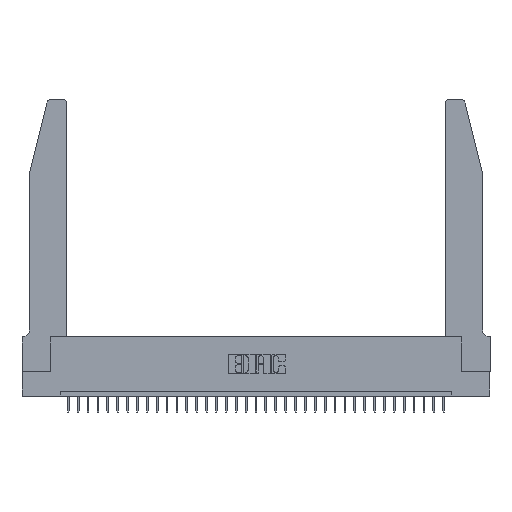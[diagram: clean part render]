
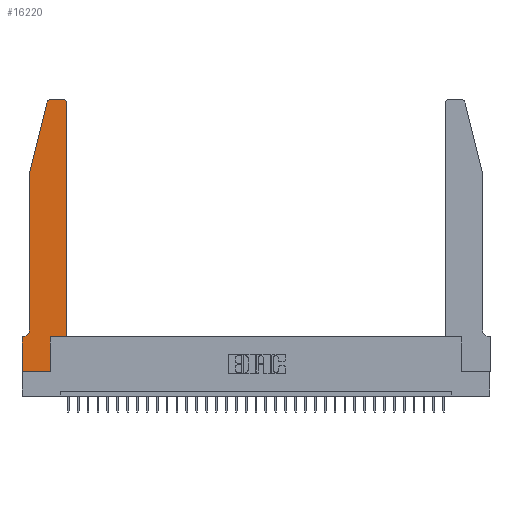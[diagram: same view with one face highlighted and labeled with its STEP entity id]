
A CAD part, top view. The second image highlights one B-rep face of the part: STEP entity #16220.
In plain terms, the highlighted planar face has unit normal (0, 0, 1).
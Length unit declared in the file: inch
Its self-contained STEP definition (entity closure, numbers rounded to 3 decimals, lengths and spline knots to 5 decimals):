
#76 = LINE ( 'NONE', #32654, #25574 ) ;
#505 = LINE ( 'NONE', #14812, #14825 ) ;
#1436 = ORIENTED_EDGE ( 'NONE', *, *, #25643, .T. ) ;
#1445 = ORIENTED_EDGE ( 'NONE', *, *, #2100, .T. ) ;
#1722 = LINE ( 'NONE', #32258, #25044 ) ;
#1838 = CARTESIAN_POINT ( 'NONE',  ( 0.0755, 0.42, 0.37 ) ) ;
#2100 = EDGE_CURVE ( 'NONE', #6404, #25170, #1722, .T. ) ;
#2389 = CIRCLE ( 'NONE', #14596, 0.03 ) ;
#2399 = CARTESIAN_POINT ( 'NONE',  ( 0.0755, 0.35, 0.37 ) ) ;
#2851 = ORIENTED_EDGE ( 'NONE', *, *, #15162, .T. ) ;
#3322 = EDGE_LOOP ( 'NONE', ( #1445, #31529, #28126, #1436, #2851, #7869, #8199, #13183, #10939, #4175, #20992, #10540 ) ) ;
#3427 = LINE ( 'NONE', #25641, #8886 ) ;
#3844 = CARTESIAN_POINT ( 'NONE',  ( 0.2865, 0., 0.37 ) ) ;
#3898 = FACE_OUTER_BOUND ( 'NONE', #3322, .T. ) ;
#4175 = ORIENTED_EDGE ( 'NONE', *, *, #10695, .T. ) ;
#4227 = DIRECTION ( 'NONE',  ( 0., -1., 0. ) ) ;
#4323 = VECTOR ( 'NONE', #4227, 39.37008 ) ;
#4511 = AXIS2_PLACEMENT_3D ( 'NONE', #9586, #7115, #20034 ) ;
#4575 = VERTEX_POINT ( 'NONE', #20891 ) ;
#6296 = CARTESIAN_POINT ( 'NONE',  ( 0.0755, 2., 0.37 ) ) ;
#6371 = VECTOR ( 'NONE', #29928, 39.37008 ) ;
#6404 = VERTEX_POINT ( 'NONE', #23749 ) ;
#7115 = DIRECTION ( 'NONE',  ( 0., 0., 1. ) ) ;
#7869 = ORIENTED_EDGE ( 'NONE', *, *, #23926, .T. ) ;
#8017 = EDGE_CURVE ( 'NONE', #28567, #26622, #76, .T. ) ;
#8063 = CARTESIAN_POINT ( 'NONE',  ( 0.4505, 0.35, 0.37 ) ) ;
#8086 = EDGE_CURVE ( 'NONE', #15128, #24139, #9329, .T. ) ;
#8184 = EDGE_CURVE ( 'NONE', #10328, #4575, #3427, .T. ) ;
#8199 = ORIENTED_EDGE ( 'NONE', *, *, #8086, .T. ) ;
#8257 = VERTEX_POINT ( 'NONE', #1838 ) ;
#8379 = CIRCLE ( 'NONE', #16040, 0.03 ) ;
#8787 = VECTOR ( 'NONE', #34493, 39.37008 ) ;
#8886 = VECTOR ( 'NONE', #15410, 39.37008 ) ;
#9039 = DIRECTION ( 'NONE',  ( 0., 0., -1. ) ) ;
#9090 = EDGE_CURVE ( 'NONE', #26622, #6404, #8379, .T. ) ;
#9329 = LINE ( 'NONE', #17511, #4323 ) ;
#9586 = CARTESIAN_POINT ( 'NONE',  ( 0., 0.35, 0.37 ) ) ;
#10328 = VERTEX_POINT ( 'NONE', #3844 ) ;
#10430 = CARTESIAN_POINT ( 'NONE',  ( 0.284, 2.75, 0.37 ) ) ;
#10540 = ORIENTED_EDGE ( 'NONE', *, *, #9090, .T. ) ;
#10667 = CIRCLE ( 'NONE', #18824, 0.07 ) ;
#10695 = EDGE_CURVE ( 'NONE', #4575, #28567, #12264, .T. ) ;
#10939 = ORIENTED_EDGE ( 'NONE', *, *, #8184, .T. ) ;
#11753 = CARTESIAN_POINT ( 'NONE',  ( 0.25487, 2.72718, 0.37 ) ) ;
#12174 = CARTESIAN_POINT ( 'NONE',  ( 0.284, 2.72, 0.37 ) ) ;
#12241 = DIRECTION ( 'NONE',  ( 1., 0., 0. ) ) ;
#12264 = LINE ( 'NONE', #8063, #6371 ) ;
#13183 = ORIENTED_EDGE ( 'NONE', *, *, #15821, .T. ) ;
#13275 = DIRECTION ( 'NONE',  ( -0.239, -0.971, 0. ) ) ;
#13540 = CARTESIAN_POINT ( 'NONE',  ( 0., 0., 0.37 ) ) ;
#13716 = EDGE_CURVE ( 'NONE', #25170, #24223, #2389, .T. ) ;
#13723 = LINE ( 'NONE', #6296, #27377 ) ;
#13868 = DIRECTION ( 'NONE',  ( 0., 0., 1. ) ) ;
#14596 = AXIS2_PLACEMENT_3D ( 'NONE', #12174, #30669, #25151 ) ;
#14812 = CARTESIAN_POINT ( 'NONE',  ( 0., 0., 0.37 ) ) ;
#14825 = VECTOR ( 'NONE', #12241, 39.37008 ) ;
#15128 = VERTEX_POINT ( 'NONE', #33172 ) ;
#15162 = EDGE_CURVE ( 'NONE', #8257, #18800, #10667, .T. ) ;
#15410 = DIRECTION ( 'NONE',  ( 0., 1., 0. ) ) ;
#15821 = EDGE_CURVE ( 'NONE', #24139, #10328, #505, .T. ) ;
#15838 = EDGE_CURVE ( 'NONE', #24223, #34137, #31050, .T. ) ;
#16040 = AXIS2_PLACEMENT_3D ( 'NONE', #29435, #13868, #16638 ) ;
#16220 = ADVANCED_FACE ( 'NONE', ( #3898 ), #23061, .T. ) ;
#16638 = DIRECTION ( 'NONE',  ( 1., 0., 0. ) ) ;
#16772 = DIRECTION ( 'NONE',  ( 0., -1., 0. ) ) ;
#17511 = CARTESIAN_POINT ( 'NONE',  ( 0., 0., 0.37 ) ) ;
#18785 = LINE ( 'NONE', #2399, #8787 ) ;
#18800 = VERTEX_POINT ( 'NONE', #33409 ) ;
#18824 = AXIS2_PLACEMENT_3D ( 'NONE', #30354, #9039, #27759 ) ;
#19197 = DIRECTION ( 'NONE',  ( 0., 1., 0. ) ) ;
#19627 = CARTESIAN_POINT ( 'NONE',  ( 0.4505, 0.35, 0.37 ) ) ;
#20034 = DIRECTION ( 'NONE',  ( 1., 0., 0. ) ) ;
#20183 = VECTOR ( 'NONE', #13275, 39.37008 ) ;
#20891 = CARTESIAN_POINT ( 'NONE',  ( 0.2865, 0.35, 0.37 ) ) ;
#20992 = ORIENTED_EDGE ( 'NONE', *, *, #8017, .T. ) ;
#22670 = CARTESIAN_POINT ( 'NONE',  ( 0.0755, 2., 0.37 ) ) ;
#23061 = PLANE ( 'NONE',  #4511 ) ;
#23749 = CARTESIAN_POINT ( 'NONE',  ( 0.4205, 2.75, 0.37 ) ) ;
#23926 = EDGE_CURVE ( 'NONE', #18800, #15128, #18785, .T. ) ;
#24139 = VERTEX_POINT ( 'NONE', #13540 ) ;
#24223 = VERTEX_POINT ( 'NONE', #11753 ) ;
#24370 = DIRECTION ( 'NONE',  ( -1., 0., 0. ) ) ;
#24483 = CARTESIAN_POINT ( 'NONE',  ( 0.4505, 2.72, 0.37 ) ) ;
#25044 = VECTOR ( 'NONE', #24370, 39.37008 ) ;
#25151 = DIRECTION ( 'NONE',  ( 1., 0., 0. ) ) ;
#25170 = VERTEX_POINT ( 'NONE', #10430 ) ;
#25574 = VECTOR ( 'NONE', #19197, 39.37008 ) ;
#25641 = CARTESIAN_POINT ( 'NONE',  ( 0.2865, 0.35, 0.37 ) ) ;
#25643 = EDGE_CURVE ( 'NONE', #34137, #8257, #13723, .T. ) ;
#26622 = VERTEX_POINT ( 'NONE', #24483 ) ;
#27377 = VECTOR ( 'NONE', #16772, 39.37008 ) ;
#27759 = DIRECTION ( 'NONE',  ( -1., 0., 0. ) ) ;
#28126 = ORIENTED_EDGE ( 'NONE', *, *, #15838, .T. ) ;
#28567 = VERTEX_POINT ( 'NONE', #19627 ) ;
#29045 = CARTESIAN_POINT ( 'NONE',  ( 0.0755, 2., 0.37 ) ) ;
#29435 = CARTESIAN_POINT ( 'NONE',  ( 0.4205, 2.72, 0.37 ) ) ;
#29928 = DIRECTION ( 'NONE',  ( 1., 0., 0. ) ) ;
#30354 = CARTESIAN_POINT ( 'NONE',  ( 0.0055, 0.42, 0.37 ) ) ;
#30669 = DIRECTION ( 'NONE',  ( 0., 0., 1. ) ) ;
#31050 = LINE ( 'NONE', #22670, #20183 ) ;
#31529 = ORIENTED_EDGE ( 'NONE', *, *, #13716, .T. ) ;
#32258 = CARTESIAN_POINT ( 'NONE',  ( 0.2605, 2.75, 0.37 ) ) ;
#32654 = CARTESIAN_POINT ( 'NONE',  ( 0.4505, 0.35, 0.37 ) ) ;
#33172 = CARTESIAN_POINT ( 'NONE',  ( 0., 0.35, 0.37 ) ) ;
#33409 = CARTESIAN_POINT ( 'NONE',  ( 0.0055, 0.35, 0.37 ) ) ;
#34137 = VERTEX_POINT ( 'NONE', #29045 ) ;
#34493 = DIRECTION ( 'NONE',  ( -1., 0., 0. ) ) ;
